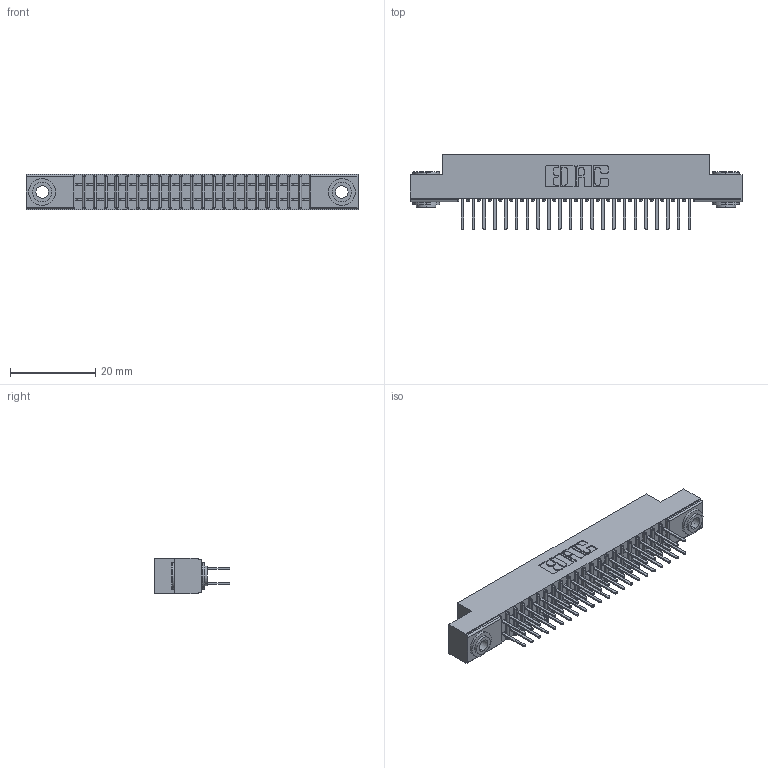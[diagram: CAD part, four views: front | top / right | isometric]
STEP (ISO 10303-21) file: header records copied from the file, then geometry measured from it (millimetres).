
FILE_DESCRIPTION (( 'STEP AP203' ), '1' );
FILE_NAME ('341-044-521-203.STEP', '2018-08-07T02:25:18', ( '' ), ( '' ), 'SwSTEP 2.0', 'SolidWorks 2016', '' );
FILE_SCHEMA (( 'CONFIG_CONTROL_DESIGN' ));
Length unit declared in the file: inch
Products named in the file (4): 345-250-002_345-250-002-102; 341-044-521-203; 341 Part_.156 (3.96) Dia Mounting Holes; 341-292-001_341-292-121
Assembly tree (47 placements, depth 2):
  341-044-521-203
    341 Part_.156 (3.96) Dia Mounting Holes
    341-292-001_341-292-121  x44
    345-250-002_345-250-002-102  x2
Bounding box: 78.11 x 17.7 x 8.38 mm (x, y, z)
Volume: 4481.3 mm3; surface area: 9760.8 mm2
Topology: 47 solids, 47 shells, 3072 faces, 8854 edges, 5734 vertices
Faces by surface type: plane 1852, cylinder 1124, sphere 46, torus 42, cone 8
Entity records: 30354 total; most frequent: CARTESIAN_POINT 5027, ORIENTED_EDGE 4984, DIRECTION 4908, EDGE_CURVE 2492, LINE 1982, VECTOR 1982, VERTEX_POINT 1582, AXIS2_PLACEMENT_3D 1463
